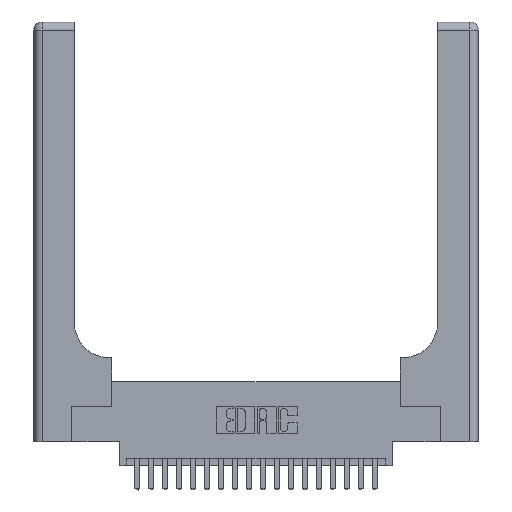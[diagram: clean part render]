
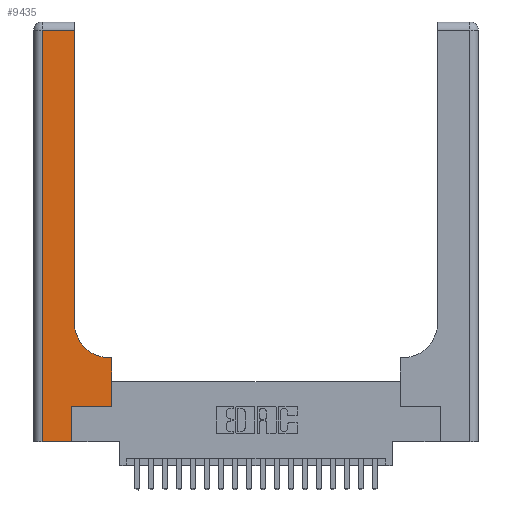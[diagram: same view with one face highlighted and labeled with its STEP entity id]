
A CAD part, top view. The second image highlights one B-rep face of the part: STEP entity #9435.
In plain terms, the highlighted planar face has unit normal (0, 0, 1).
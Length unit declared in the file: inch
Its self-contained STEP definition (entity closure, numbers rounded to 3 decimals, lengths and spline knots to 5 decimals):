
#344 = DIRECTION ( 'NONE',  ( 0., -1., 0. ) ) ;
#659 = DIRECTION ( 'NONE',  ( -1., 0., 0. ) ) ;
#875 = CIRCLE ( 'NONE', #10969, 0.25 ) ;
#2611 = VECTOR ( 'NONE', #18250, 39.37008 ) ;
#2824 = VECTOR ( 'NONE', #344, 39.37008 ) ;
#2854 = CARTESIAN_POINT ( 'NONE',  ( 0.269, 0.25, 0.37 ) ) ;
#3027 = AXIS2_PLACEMENT_3D ( 'NONE', #6019, #21795, #18393 ) ;
#3494 = CARTESIAN_POINT ( 'NONE',  ( 0.2915, 0.85, 0.37 ) ) ;
#3911 = ORIENTED_EDGE ( 'NONE', *, *, #4325, .T. ) ;
#3950 = ORIENTED_EDGE ( 'NONE', *, *, #5816, .T. ) ;
#4048 = ORIENTED_EDGE ( 'NONE', *, *, #15245, .T. ) ;
#4282 = ORIENTED_EDGE ( 'NONE', *, *, #10185, .T. ) ;
#4284 = VERTEX_POINT ( 'NONE', #2854 ) ;
#4325 = EDGE_CURVE ( 'NONE', #19711, #4284, #17911, .T. ) ;
#4461 = CARTESIAN_POINT ( 'NONE',  ( 0.269, 0., 0.37 ) ) ;
#4740 = LINE ( 'NONE', #11306, #20117 ) ;
#4741 = ORIENTED_EDGE ( 'NONE', *, *, #8002, .T. ) ;
#4988 = CARTESIAN_POINT ( 'NONE',  ( 0.269, 0., 0.37 ) ) ;
#5313 = ORIENTED_EDGE ( 'NONE', *, *, #15127, .T. ) ;
#5729 = DIRECTION ( 'NONE',  ( 0., 0., -1. ) ) ;
#5776 = CARTESIAN_POINT ( 'NONE',  ( 0.5585, 0.25, 0.37 ) ) ;
#5816 = EDGE_CURVE ( 'NONE', #21593, #22503, #7431, .T. ) ;
#6019 = CARTESIAN_POINT ( 'NONE',  ( 0., 3., 0.37 ) ) ;
#6291 = VECTOR ( 'NONE', #10349, 39.37008 ) ;
#6307 = PLANE ( 'NONE',  #3027 ) ;
#6902 = VECTOR ( 'NONE', #659, 39.37008 ) ;
#6963 = CARTESIAN_POINT ( 'NONE',  ( 0.5585, 0.25, 0.37 ) ) ;
#7076 = EDGE_CURVE ( 'NONE', #13768, #21593, #10958, .T. ) ;
#7431 = LINE ( 'NONE', #19825, #6902 ) ;
#8002 = EDGE_CURVE ( 'NONE', #17062, #9697, #12862, .T. ) ;
#8835 = CARTESIAN_POINT ( 'NONE',  ( 0.5415, 0.6, 0.37 ) ) ;
#9089 = VECTOR ( 'NONE', #14826, 39.37008 ) ;
#9294 = EDGE_CURVE ( 'NONE', #4284, #17062, #15264, .T. ) ;
#9383 = CARTESIAN_POINT ( 'NONE',  ( 0.269, 0.25, 0.37 ) ) ;
#9435 = ADVANCED_FACE ( 'NONE', ( #20494 ), #6307, .F. ) ;
#9697 = VERTEX_POINT ( 'NONE', #22573 ) ;
#10185 = EDGE_CURVE ( 'NONE', #13236, #19711, #12204, .T. ) ;
#10349 = DIRECTION ( 'NONE',  ( 0., 1., 0. ) ) ;
#10625 = CARTESIAN_POINT ( 'NONE',  ( 0.06, 0., 0.37 ) ) ;
#10919 = EDGE_CURVE ( 'NONE', #13804, #13768, #875, .T. ) ;
#10958 = LINE ( 'NONE', #15584, #6291 ) ;
#10969 = AXIS2_PLACEMENT_3D ( 'NONE', #19806, #5729, #14514 ) ;
#11306 = CARTESIAN_POINT ( 'NONE',  ( 0.2915, 0.6, 0.37 ) ) ;
#12204 = LINE ( 'NONE', #19732, #14951 ) ;
#12342 = DIRECTION ( 'NONE',  ( 1., 0., 0. ) ) ;
#12862 = LINE ( 'NONE', #5776, #20562 ) ;
#12870 = CARTESIAN_POINT ( 'NONE',  ( 0.06, 3., 0.37 ) ) ;
#13236 = VERTEX_POINT ( 'NONE', #10625 ) ;
#13768 = VERTEX_POINT ( 'NONE', #3494 ) ;
#13804 = VERTEX_POINT ( 'NONE', #8835 ) ;
#13809 = ORIENTED_EDGE ( 'NONE', *, *, #10919, .T. ) ;
#14514 = DIRECTION ( 'NONE',  ( 1., 0., 0. ) ) ;
#14826 = DIRECTION ( 'NONE',  ( 0., 1., 0. ) ) ;
#14951 = VECTOR ( 'NONE', #12342, 39.37008 ) ;
#15127 = EDGE_CURVE ( 'NONE', #22503, #13236, #16827, .T. ) ;
#15163 = ORIENTED_EDGE ( 'NONE', *, *, #9294, .T. ) ;
#15245 = EDGE_CURVE ( 'NONE', #9697, #13804, #4740, .T. ) ;
#15264 = LINE ( 'NONE', #9383, #2611 ) ;
#15584 = CARTESIAN_POINT ( 'NONE',  ( 0.2915, 3., 0.37 ) ) ;
#15806 = ORIENTED_EDGE ( 'NONE', *, *, #7076, .T. ) ;
#16543 = DIRECTION ( 'NONE',  ( -1., 0., 0. ) ) ;
#16689 = EDGE_LOOP ( 'NONE', ( #15806, #3950, #5313, #4282, #3911, #15163, #4741, #4048, #13809 ) ) ;
#16827 = LINE ( 'NONE', #12870, #2824 ) ;
#17062 = VERTEX_POINT ( 'NONE', #6963 ) ;
#17911 = LINE ( 'NONE', #4461, #9089 ) ;
#18250 = DIRECTION ( 'NONE',  ( 1., 0., 0. ) ) ;
#18393 = DIRECTION ( 'NONE',  ( -1., 0., 0. ) ) ;
#18971 = CARTESIAN_POINT ( 'NONE',  ( 0.2915, 2.94, 0.37 ) ) ;
#19711 = VERTEX_POINT ( 'NONE', #4988 ) ;
#19732 = CARTESIAN_POINT ( 'NONE',  ( 0., 0., 0.37 ) ) ;
#19806 = CARTESIAN_POINT ( 'NONE',  ( 0.5415, 0.85, 0.37 ) ) ;
#19825 = CARTESIAN_POINT ( 'NONE',  ( 0., 2.94, 0.37 ) ) ;
#20117 = VECTOR ( 'NONE', #16543, 39.37008 ) ;
#20494 = FACE_OUTER_BOUND ( 'NONE', #16689, .T. ) ;
#20562 = VECTOR ( 'NONE', #21622, 39.37008 ) ;
#20872 = CARTESIAN_POINT ( 'NONE',  ( 0.06, 2.94, 0.37 ) ) ;
#21593 = VERTEX_POINT ( 'NONE', #18971 ) ;
#21622 = DIRECTION ( 'NONE',  ( 0., 1., 0. ) ) ;
#21795 = DIRECTION ( 'NONE',  ( 0., 0., -1. ) ) ;
#22503 = VERTEX_POINT ( 'NONE', #20872 ) ;
#22573 = CARTESIAN_POINT ( 'NONE',  ( 0.5585, 0.6, 0.37 ) ) ;
